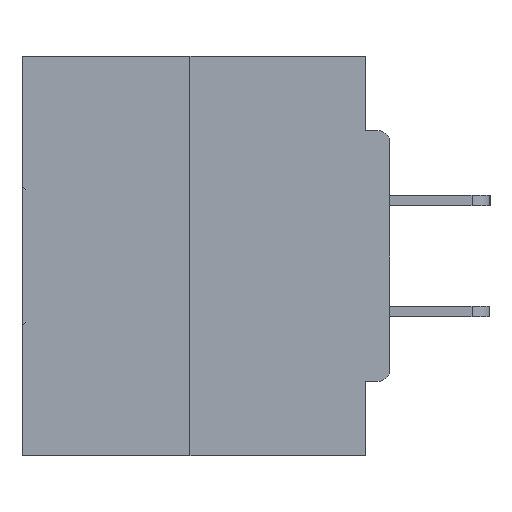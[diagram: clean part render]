
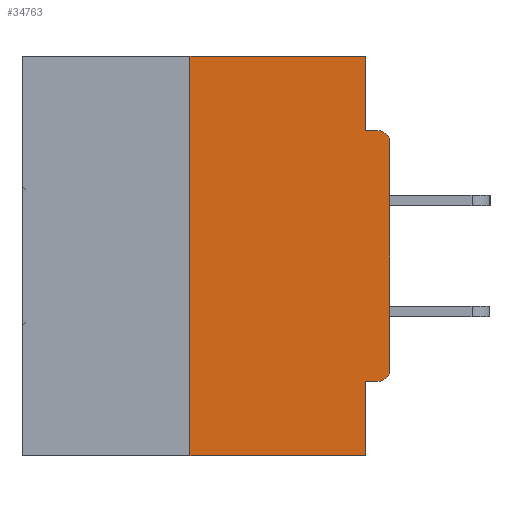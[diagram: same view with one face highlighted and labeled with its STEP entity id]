
A CAD part, left-side view. The second image highlights one B-rep face of the part: STEP entity #34763.
In plain terms, the highlighted planar face has unit normal (-1, 0, 0).
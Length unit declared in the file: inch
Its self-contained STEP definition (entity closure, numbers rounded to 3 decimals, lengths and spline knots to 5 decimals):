
#283 = CARTESIAN_POINT ( 'NONE',  ( 0., 0., -0.4065 ) ) ;
#511 = DIRECTION ( 'NONE',  ( -1., 0., 0. ) ) ;
#759 = VECTOR ( 'NONE', #27544, 39.37008 ) ;
#1926 = ORIENTED_EDGE ( 'NONE', *, *, #18661, .F. ) ;
#2493 = DIRECTION ( 'NONE',  ( 0., -1., 0. ) ) ;
#2621 = DIRECTION ( 'NONE',  ( 0., 0., -1. ) ) ;
#2669 = LINE ( 'NONE', #22681, #36439 ) ;
#3257 = CIRCLE ( 'NONE', #13725, 0.015 ) ;
#4554 = EDGE_CURVE ( 'NONE', #29912, #33737, #9304, .T. ) ;
#4636 = EDGE_CURVE ( 'NONE', #42599, #19865, #43471, .T. ) ;
#5191 = AXIS2_PLACEMENT_3D ( 'NONE', #9669, #29635, #23138 ) ;
#5545 = CARTESIAN_POINT ( 'NONE',  ( 0., 0.46, 0. ) ) ;
#5884 = CARTESIAN_POINT ( 'NONE',  ( 0., 0., 0. ) ) ;
#6068 = DIRECTION ( 'NONE',  ( 0., 0., -1. ) ) ;
#6630 = EDGE_CURVE ( 'NONE', #15945, #23995, #3257, .T. ) ;
#9304 = CIRCLE ( 'NONE', #5191, 0.015 ) ;
#9454 = DIRECTION ( 'NONE',  ( 0., 0., 1. ) ) ;
#9523 = ORIENTED_EDGE ( 'NONE', *, *, #28778, .F. ) ;
#9530 = FACE_OUTER_BOUND ( 'NONE', #30012, .T. ) ;
#9669 = CARTESIAN_POINT ( 'NONE',  ( 0., 0.015, -0.1085 ) ) ;
#9734 = PLANE ( 'NONE',  #28730 ) ;
#10073 = CARTESIAN_POINT ( 'NONE',  ( 0., 0.031, 0. ) ) ;
#10925 = LINE ( 'NONE', #5545, #33059 ) ;
#10996 = CARTESIAN_POINT ( 'NONE',  ( 0., 0., -0.1085 ) ) ;
#11347 = CARTESIAN_POINT ( 'NONE',  ( 0., 0., -0.0935 ) ) ;
#11945 = DIRECTION ( 'NONE',  ( 0., -1., 0. ) ) ;
#12343 = LINE ( 'NONE', #283, #34457 ) ;
#13119 = DIRECTION ( 'NONE',  ( 0., 0., -1. ) ) ;
#13366 = EDGE_CURVE ( 'NONE', #42914, #22584, #20111, .T. ) ;
#13725 = AXIS2_PLACEMENT_3D ( 'NONE', #37221, #511, #34145 ) ;
#13743 = CARTESIAN_POINT ( 'NONE',  ( 0., 0.031, -0.4065 ) ) ;
#14800 = CARTESIAN_POINT ( 'NONE',  ( 0., 0.031, -0.0935 ) ) ;
#15573 = LINE ( 'NONE', #11347, #26541 ) ;
#15689 = CARTESIAN_POINT ( 'NONE',  ( 0., 0.25, 0. ) ) ;
#15945 = VERTEX_POINT ( 'NONE', #20412 ) ;
#16498 = ORIENTED_EDGE ( 'NONE', *, *, #38874, .F. ) ;
#18148 = EDGE_CURVE ( 'NONE', #23995, #29912, #31410, .T. ) ;
#18228 = DIRECTION ( 'NONE',  ( 0., -1., 0. ) ) ;
#18661 = EDGE_CURVE ( 'NONE', #42979, #33737, #15573, .T. ) ;
#19847 = DIRECTION ( 'NONE',  ( 1., 0., 0. ) ) ;
#19865 = VERTEX_POINT ( 'NONE', #15689 ) ;
#20111 = LINE ( 'NONE', #26068, #25900 ) ;
#20412 = CARTESIAN_POINT ( 'NONE',  ( 0., 0.015, -0.4065 ) ) ;
#20465 = DIRECTION ( 'NONE',  ( 0., 1., 0. ) ) ;
#20690 = CARTESIAN_POINT ( 'NONE',  ( 0., 0.031, -0.5 ) ) ;
#22584 = VERTEX_POINT ( 'NONE', #20690 ) ;
#22681 = CARTESIAN_POINT ( 'NONE',  ( 0., 0.46, -0.5 ) ) ;
#23093 = ORIENTED_EDGE ( 'NONE', *, *, #4554, .T. ) ;
#23138 = DIRECTION ( 'NONE',  ( 0., 0., -1. ) ) ;
#23995 = VERTEX_POINT ( 'NONE', #43080 ) ;
#25900 = VECTOR ( 'NONE', #6068, 39.37008 ) ;
#26068 = CARTESIAN_POINT ( 'NONE',  ( 0., 0.031, -0.5 ) ) ;
#26072 = EDGE_CURVE ( 'NONE', #26196, #42979, #40346, .T. ) ;
#26196 = VERTEX_POINT ( 'NONE', #10073 ) ;
#26541 = VECTOR ( 'NONE', #18228, 39.37008 ) ;
#27255 = CARTESIAN_POINT ( 'NONE',  ( 0., 0.25, 0. ) ) ;
#27544 = DIRECTION ( 'NONE',  ( 0., 0., 1. ) ) ;
#27666 = CARTESIAN_POINT ( 'NONE',  ( 0., 0.015, -0.0935 ) ) ;
#28730 = AXIS2_PLACEMENT_3D ( 'NONE', #40286, #19847, #13119 ) ;
#28778 = EDGE_CURVE ( 'NONE', #19865, #26196, #10925, .T. ) ;
#29093 = ORIENTED_EDGE ( 'NONE', *, *, #26072, .F. ) ;
#29635 = DIRECTION ( 'NONE',  ( -1., 0., 0. ) ) ;
#29912 = VERTEX_POINT ( 'NONE', #10996 ) ;
#30012 = EDGE_LOOP ( 'NONE', ( #9523, #32430, #32785, #33605, #16498, #31995, #42239, #23093, #1926, #29093 ) ) ;
#31410 = LINE ( 'NONE', #5884, #37139 ) ;
#31431 = VECTOR ( 'NONE', #2621, 39.37008 ) ;
#31995 = ORIENTED_EDGE ( 'NONE', *, *, #6630, .T. ) ;
#32409 = EDGE_CURVE ( 'NONE', #42599, #22584, #2669, .T. ) ;
#32430 = ORIENTED_EDGE ( 'NONE', *, *, #4636, .F. ) ;
#32785 = ORIENTED_EDGE ( 'NONE', *, *, #32409, .T. ) ;
#32875 = CARTESIAN_POINT ( 'NONE',  ( 0., 0.031, 0. ) ) ;
#33059 = VECTOR ( 'NONE', #11945, 39.37008 ) ;
#33605 = ORIENTED_EDGE ( 'NONE', *, *, #13366, .F. ) ;
#33737 = VERTEX_POINT ( 'NONE', #27666 ) ;
#34145 = DIRECTION ( 'NONE',  ( 0., 0., -1. ) ) ;
#34457 = VECTOR ( 'NONE', #20465, 39.37008 ) ;
#34763 = ADVANCED_FACE ( 'NONE', ( #9530 ), #9734, .F. ) ;
#36439 = VECTOR ( 'NONE', #2493, 39.37008 ) ;
#37139 = VECTOR ( 'NONE', #9454, 39.37008 ) ;
#37221 = CARTESIAN_POINT ( 'NONE',  ( 0., 0.015, -0.3915 ) ) ;
#38874 = EDGE_CURVE ( 'NONE', #15945, #42914, #12343, .T. ) ;
#40286 = CARTESIAN_POINT ( 'NONE',  ( 0., 0.46, 0. ) ) ;
#40346 = LINE ( 'NONE', #32875, #31431 ) ;
#40540 = CARTESIAN_POINT ( 'NONE',  ( 0., 0.25, -0.5 ) ) ;
#42239 = ORIENTED_EDGE ( 'NONE', *, *, #18148, .T. ) ;
#42599 = VERTEX_POINT ( 'NONE', #40540 ) ;
#42914 = VERTEX_POINT ( 'NONE', #13743 ) ;
#42979 = VERTEX_POINT ( 'NONE', #14800 ) ;
#43080 = CARTESIAN_POINT ( 'NONE',  ( 0., 0., -0.3915 ) ) ;
#43471 = LINE ( 'NONE', #27255, #759 ) ;
